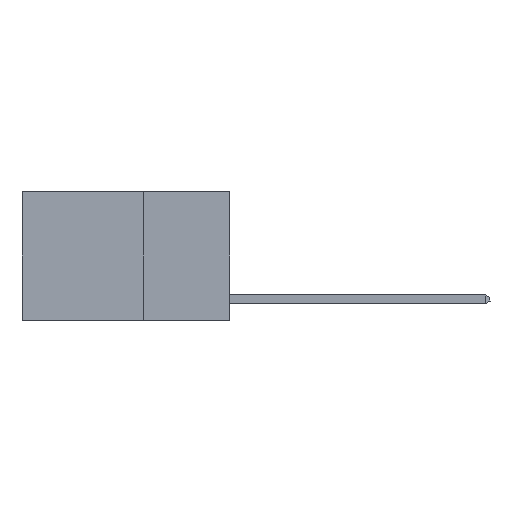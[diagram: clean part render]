
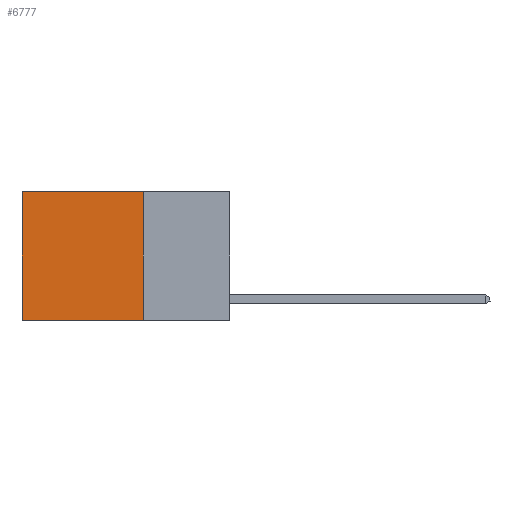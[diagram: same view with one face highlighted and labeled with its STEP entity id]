
A CAD part, left-side view. The second image highlights one B-rep face of the part: STEP entity #6777.
In plain terms, the highlighted planar face has unit normal (-1, 0, 0).
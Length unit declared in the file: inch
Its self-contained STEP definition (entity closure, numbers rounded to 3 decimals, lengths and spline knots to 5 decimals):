
#155 = ORIENTED_EDGE ( 'NONE', *, *, #9575, .F. ) ;
#418 = VERTEX_POINT ( 'NONE', #21775 ) ;
#1483 = EDGE_CURVE ( 'NONE', #4933, #418, #21227, .T. ) ;
#2162 = DIRECTION ( 'NONE',  ( 0., 0., -1. ) ) ;
#2227 = DIRECTION ( 'NONE',  ( 0., 1., 0. ) ) ;
#2712 = FACE_OUTER_BOUND ( 'NONE', #17504, .T. ) ;
#2923 = CARTESIAN_POINT ( 'NONE',  ( 0.2625, 0.6, 0. ) ) ;
#3656 = VECTOR ( 'NONE', #23675, 39.37008 ) ;
#3971 = LINE ( 'NONE', #7872, #23500 ) ;
#4556 = EDGE_CURVE ( 'NONE', #8268, #14605, #3971, .T. ) ;
#4933 = VERTEX_POINT ( 'NONE', #24147 ) ;
#5242 = CARTESIAN_POINT ( 'NONE',  ( 0.2625, 0.25, 0. ) ) ;
#5858 = ORIENTED_EDGE ( 'NONE', *, *, #4556, .T. ) ;
#5882 = LINE ( 'NONE', #9717, #15368 ) ;
#6777 = ADVANCED_FACE ( 'NONE', ( #2712 ), #16616, .F. ) ;
#7137 = DIRECTION ( 'NONE',  ( 1., 0., 0. ) ) ;
#7872 = CARTESIAN_POINT ( 'NONE',  ( 0.2625, 0.25, 0. ) ) ;
#8268 = VERTEX_POINT ( 'NONE', #17042 ) ;
#9575 = EDGE_CURVE ( 'NONE', #8268, #4933, #5882, .T. ) ;
#9717 = CARTESIAN_POINT ( 'NONE',  ( 0.2625, 0.25, 0. ) ) ;
#10869 = DIRECTION ( 'NONE',  ( 0., 1., 0. ) ) ;
#11183 = VECTOR ( 'NONE', #10869, 39.37008 ) ;
#11362 = CARTESIAN_POINT ( 'NONE',  ( 0.2625, 0.6, 0. ) ) ;
#12210 = EDGE_CURVE ( 'NONE', #14605, #418, #14364, .T. ) ;
#12272 = AXIS2_PLACEMENT_3D ( 'NONE', #5242, #7137, #20370 ) ;
#14364 = LINE ( 'NONE', #2923, #3656 ) ;
#14605 = VERTEX_POINT ( 'NONE', #11362 ) ;
#15368 = VECTOR ( 'NONE', #2162, 39.37008 ) ;
#15829 = ORIENTED_EDGE ( 'NONE', *, *, #12210, .T. ) ;
#16616 = PLANE ( 'NONE',  #12272 ) ;
#17042 = CARTESIAN_POINT ( 'NONE',  ( 0.2625, 0.25, 0. ) ) ;
#17504 = EDGE_LOOP ( 'NONE', ( #15829, #22161, #155, #5858 ) ) ;
#20370 = DIRECTION ( 'NONE',  ( 0., 0., -1. ) ) ;
#21227 = LINE ( 'NONE', #22204, #11183 ) ;
#21775 = CARTESIAN_POINT ( 'NONE',  ( 0.2625, 0.6, -0.37 ) ) ;
#22161 = ORIENTED_EDGE ( 'NONE', *, *, #1483, .F. ) ;
#22204 = CARTESIAN_POINT ( 'NONE',  ( 0.2625, 0.25, -0.37 ) ) ;
#23500 = VECTOR ( 'NONE', #2227, 39.37008 ) ;
#23675 = DIRECTION ( 'NONE',  ( 0., 0., -1. ) ) ;
#24147 = CARTESIAN_POINT ( 'NONE',  ( 0.2625, 0.25, -0.37 ) ) ;
